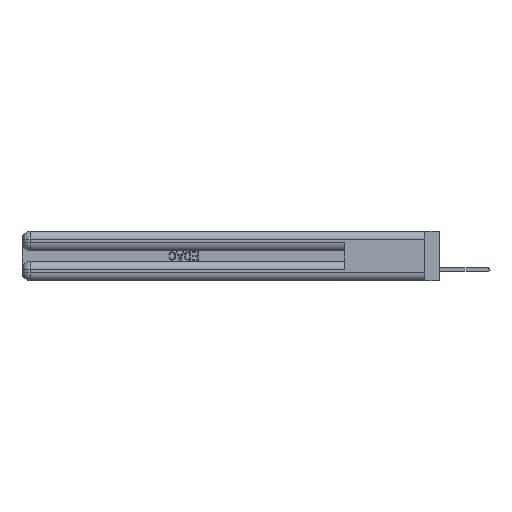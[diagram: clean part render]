
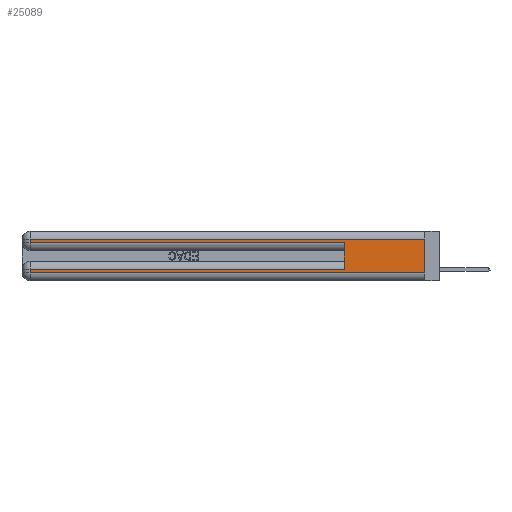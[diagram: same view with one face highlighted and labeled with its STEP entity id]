
A CAD part, left-side view. The second image highlights one B-rep face of the part: STEP entity #25089.
In plain terms, the highlighted planar face has unit normal (-1, 0, 0).
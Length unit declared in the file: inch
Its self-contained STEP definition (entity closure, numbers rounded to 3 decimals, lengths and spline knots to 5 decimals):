
#1909 = EDGE_CURVE ( 'NONE', #13310, #25607, #3736, .T. ) ;
#2943 = CARTESIAN_POINT ( 'NONE',  ( 0., 0.6, 0.285 ) ) ;
#2957 = CARTESIAN_POINT ( 'NONE',  ( 0., 0.6, 0.085 ) ) ;
#3736 = LINE ( 'NONE', #29221, #39631 ) ;
#3758 = CARTESIAN_POINT ( 'NONE',  ( 0., 2.94, 0.285 ) ) ;
#3834 = LINE ( 'NONE', #9781, #32714 ) ;
#5126 = DIRECTION ( 'NONE',  ( 1., 0., 0. ) ) ;
#5541 = PLANE ( 'NONE',  #25634 ) ;
#6823 = FACE_OUTER_BOUND ( 'NONE', #27819, .T. ) ;
#7359 = ORIENTED_EDGE ( 'NONE', *, *, #21521, .T. ) ;
#8147 = EDGE_CURVE ( 'NONE', #9376, #18997, #30603, .T. ) ;
#9376 = VERTEX_POINT ( 'NONE', #2957 ) ;
#9710 = DIRECTION ( 'NONE',  ( 0., 0., -1. ) ) ;
#9781 = CARTESIAN_POINT ( 'NONE',  ( 0., 0.6, 0.145 ) ) ;
#10053 = DIRECTION ( 'NONE',  ( 0., -1., 0. ) ) ;
#10843 = LINE ( 'NONE', #11895, #39087 ) ;
#11113 = LINE ( 'NONE', #17805, #29990 ) ;
#11216 = VECTOR ( 'NONE', #10053, 39.37008 ) ;
#11895 = CARTESIAN_POINT ( 'NONE',  ( 0., 0., 0.37 ) ) ;
#12881 = DIRECTION ( 'NONE',  ( 0., 0., -1. ) ) ;
#13310 = VERTEX_POINT ( 'NONE', #39109 ) ;
#13497 = VECTOR ( 'NONE', #24077, 39.37008 ) ;
#13629 = DIRECTION ( 'NONE',  ( 0., 0., -1. ) ) ;
#13632 = CARTESIAN_POINT ( 'NONE',  ( 0., 2.94, 0.06 ) ) ;
#14427 = ORIENTED_EDGE ( 'NONE', *, *, #1909, .T. ) ;
#14743 = EDGE_CURVE ( 'NONE', #9376, #15142, #3834, .T. ) ;
#15085 = DIRECTION ( 'NONE',  ( 0., 0., -1. ) ) ;
#15142 = VERTEX_POINT ( 'NONE', #2943 ) ;
#15179 = VECTOR ( 'NONE', #24448, 39.37008 ) ;
#15720 = LINE ( 'NONE', #24291, #15179 ) ;
#16996 = CARTESIAN_POINT ( 'NONE',  ( 0., 0., 0.285 ) ) ;
#17042 = VERTEX_POINT ( 'NONE', #17223 ) ;
#17223 = CARTESIAN_POINT ( 'NONE',  ( 0., 0., 0.06 ) ) ;
#17805 = CARTESIAN_POINT ( 'NONE',  ( 0., 2.94, 0.37 ) ) ;
#18027 = DIRECTION ( 'NONE',  ( 0., 0., 1. ) ) ;
#18263 = ORIENTED_EDGE ( 'NONE', *, *, #27886, .T. ) ;
#18997 = VERTEX_POINT ( 'NONE', #22691 ) ;
#21521 = EDGE_CURVE ( 'NONE', #46824, #15142, #28964, .T. ) ;
#22676 = LINE ( 'NONE', #28648, #33828 ) ;
#22691 = CARTESIAN_POINT ( 'NONE',  ( 0., 2.94, 0.085 ) ) ;
#23822 = ORIENTED_EDGE ( 'NONE', *, *, #47000, .F. ) ;
#24077 = DIRECTION ( 'NONE',  ( 0., 1., 0. ) ) ;
#24291 = CARTESIAN_POINT ( 'NONE',  ( 0., 0., 0.06 ) ) ;
#24448 = DIRECTION ( 'NONE',  ( 0., -1., 0. ) ) ;
#24667 = VERTEX_POINT ( 'NONE', #13632 ) ;
#25089 = ADVANCED_FACE ( 'NONE', ( #6823 ), #5541, .F. ) ;
#25607 = VERTEX_POINT ( 'NONE', #38628 ) ;
#25634 = AXIS2_PLACEMENT_3D ( 'NONE', #26565, #5126, #15085 ) ;
#26565 = CARTESIAN_POINT ( 'NONE',  ( 0., 0., 0.37 ) ) ;
#27445 = EDGE_CURVE ( 'NONE', #25607, #46824, #22676, .T. ) ;
#27819 = EDGE_LOOP ( 'NONE', ( #23822, #14427, #41961, #7359, #31426, #31478, #18263, #45268 ) ) ;
#27886 = EDGE_CURVE ( 'NONE', #18997, #24667, #11113, .T. ) ;
#28648 = CARTESIAN_POINT ( 'NONE',  ( 0., 2.94, 0.37 ) ) ;
#28964 = LINE ( 'NONE', #16996, #11216 ) ;
#29221 = CARTESIAN_POINT ( 'NONE',  ( 0., 0., 0.31 ) ) ;
#29990 = VECTOR ( 'NONE', #9710, 39.37008 ) ;
#30603 = LINE ( 'NONE', #34899, #13497 ) ;
#31426 = ORIENTED_EDGE ( 'NONE', *, *, #14743, .F. ) ;
#31478 = ORIENTED_EDGE ( 'NONE', *, *, #8147, .T. ) ;
#32351 = DIRECTION ( 'NONE',  ( 0., 1., 0. ) ) ;
#32714 = VECTOR ( 'NONE', #18027, 39.37008 ) ;
#33828 = VECTOR ( 'NONE', #13629, 39.37008 ) ;
#34899 = CARTESIAN_POINT ( 'NONE',  ( 0., 0., 0.085 ) ) ;
#38628 = CARTESIAN_POINT ( 'NONE',  ( 0., 2.94, 0.31 ) ) ;
#38642 = EDGE_CURVE ( 'NONE', #24667, #17042, #15720, .T. ) ;
#39087 = VECTOR ( 'NONE', #12881, 39.37008 ) ;
#39109 = CARTESIAN_POINT ( 'NONE',  ( 0., 0., 0.31 ) ) ;
#39631 = VECTOR ( 'NONE', #32351, 39.37008 ) ;
#41961 = ORIENTED_EDGE ( 'NONE', *, *, #27445, .T. ) ;
#45268 = ORIENTED_EDGE ( 'NONE', *, *, #38642, .T. ) ;
#46824 = VERTEX_POINT ( 'NONE', #3758 ) ;
#47000 = EDGE_CURVE ( 'NONE', #13310, #17042, #10843, .T. ) ;
